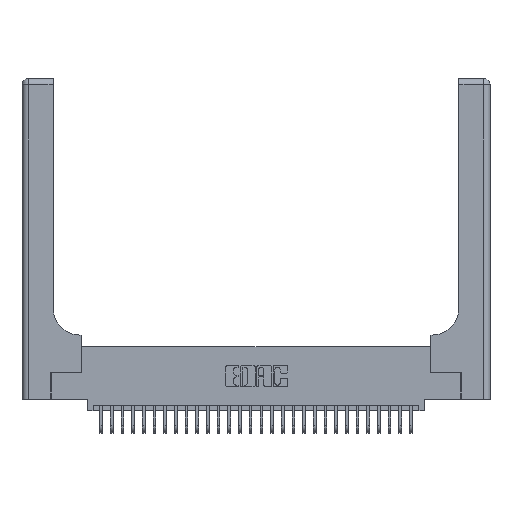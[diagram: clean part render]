
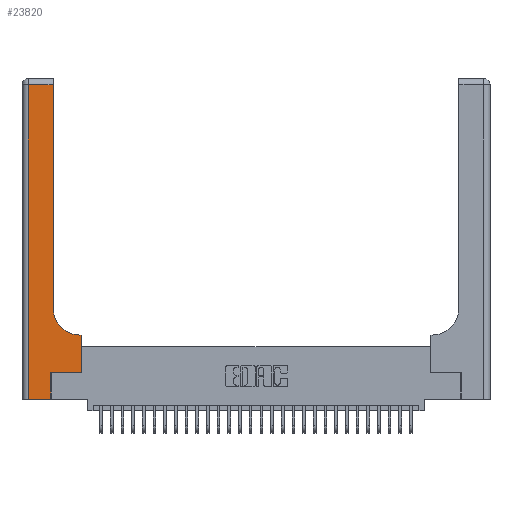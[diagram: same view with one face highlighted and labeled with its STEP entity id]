
A CAD part, top view. The second image highlights one B-rep face of the part: STEP entity #23820.
In plain terms, the highlighted planar face has unit normal (0, 0, 1).
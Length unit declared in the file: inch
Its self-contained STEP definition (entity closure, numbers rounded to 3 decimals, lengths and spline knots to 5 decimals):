
#377 = AXIS2_PLACEMENT_3D ( 'NONE', #19312, #4376, #21785 ) ;
#1062 = EDGE_CURVE ( 'NONE', #21715, #22190, #10786, .T. ) ;
#1196 = VECTOR ( 'NONE', #5113, 39.37008 ) ;
#1366 = EDGE_CURVE ( 'NONE', #31991, #13463, #16976, .T. ) ;
#1602 = CARTESIAN_POINT ( 'NONE',  ( 0.5415, 0.6, 0.37 ) ) ;
#2216 = VERTEX_POINT ( 'NONE', #30180 ) ;
#3138 = ORIENTED_EDGE ( 'NONE', *, *, #14814, .T. ) ;
#3196 = LINE ( 'NONE', #15899, #11464 ) ;
#3696 = VECTOR ( 'NONE', #29166, 39.37008 ) ;
#4099 = VECTOR ( 'NONE', #30759, 39.37008 ) ;
#4188 = EDGE_LOOP ( 'NONE', ( #12553, #32121, #7491, #20711, #28719, #3138, #16432, #11417, #30984 ) ) ;
#4376 = DIRECTION ( 'NONE',  ( 0., 0., -1. ) ) ;
#5113 = DIRECTION ( 'NONE',  ( -1., 0., 0. ) ) ;
#5179 = LINE ( 'NONE', #13146, #16843 ) ;
#6065 = DIRECTION ( 'NONE',  ( 1., 0., 0. ) ) ;
#6357 = CARTESIAN_POINT ( 'NONE',  ( 0.5585, 0.6, 0.37 ) ) ;
#7491 = ORIENTED_EDGE ( 'NONE', *, *, #1062, .T. ) ;
#7966 = LINE ( 'NONE', #27280, #1196 ) ;
#8907 = CARTESIAN_POINT ( 'NONE',  ( 0.2915, 2.94, 0.37 ) ) ;
#10083 = CARTESIAN_POINT ( 'NONE',  ( 0., 3., 0.37 ) ) ;
#10786 = LINE ( 'NONE', #13496, #4099 ) ;
#10850 = CARTESIAN_POINT ( 'NONE',  ( 0.5585, 0.25, 0.37 ) ) ;
#10950 = CARTESIAN_POINT ( 'NONE',  ( 0.2915, 3., 0.37 ) ) ;
#11417 = ORIENTED_EDGE ( 'NONE', *, *, #29906, .T. ) ;
#11464 = VECTOR ( 'NONE', #30570, 39.37008 ) ;
#11958 = CARTESIAN_POINT ( 'NONE',  ( 0.5585, 0.25, 0.37 ) ) ;
#12038 = EDGE_CURVE ( 'NONE', #2216, #28233, #3196, .T. ) ;
#12553 = ORIENTED_EDGE ( 'NONE', *, *, #23826, .T. ) ;
#12583 = DIRECTION ( 'NONE',  ( 0., 0., -1. ) ) ;
#12895 = VERTEX_POINT ( 'NONE', #1602 ) ;
#13128 = FACE_OUTER_BOUND ( 'NONE', #4188, .T. ) ;
#13146 = CARTESIAN_POINT ( 'NONE',  ( 0.269, 0.25, 0.37 ) ) ;
#13463 = VERTEX_POINT ( 'NONE', #6357 ) ;
#13496 = CARTESIAN_POINT ( 'NONE',  ( 0.06, 3., 0.37 ) ) ;
#13615 = CARTESIAN_POINT ( 'NONE',  ( 0., 2.94, 0.37 ) ) ;
#14814 = EDGE_CURVE ( 'NONE', #28233, #31991, #5179, .T. ) ;
#15082 = DIRECTION ( 'NONE',  ( 0., 1., 0. ) ) ;
#15899 = CARTESIAN_POINT ( 'NONE',  ( 0.269, 0., 0.37 ) ) ;
#16101 = DIRECTION ( 'NONE',  ( -1., 0., 0. ) ) ;
#16432 = ORIENTED_EDGE ( 'NONE', *, *, #1366, .T. ) ;
#16533 = VECTOR ( 'NONE', #16101, 39.37008 ) ;
#16843 = VECTOR ( 'NONE', #20636, 39.37008 ) ;
#16976 = LINE ( 'NONE', #11958, #3696 ) ;
#16995 = CARTESIAN_POINT ( 'NONE',  ( 0.06, 2.94, 0.37 ) ) ;
#17264 = CARTESIAN_POINT ( 'NONE',  ( 0.2915, 0.85, 0.37 ) ) ;
#18191 = VECTOR ( 'NONE', #6065, 39.37008 ) ;
#18557 = CARTESIAN_POINT ( 'NONE',  ( 0., 0., 0.37 ) ) ;
#19312 = CARTESIAN_POINT ( 'NONE',  ( 0.5415, 0.85, 0.37 ) ) ;
#19432 = CIRCLE ( 'NONE', #377, 0.25 ) ;
#19739 = LINE ( 'NONE', #10950, #25460 ) ;
#20230 = EDGE_CURVE ( 'NONE', #21026, #21715, #27308, .T. ) ;
#20636 = DIRECTION ( 'NONE',  ( 1., 0., 0. ) ) ;
#20711 = ORIENTED_EDGE ( 'NONE', *, *, #23418, .T. ) ;
#21026 = VERTEX_POINT ( 'NONE', #8907 ) ;
#21715 = VERTEX_POINT ( 'NONE', #16995 ) ;
#21785 = DIRECTION ( 'NONE',  ( 1., 0., 0. ) ) ;
#22190 = VERTEX_POINT ( 'NONE', #26207 ) ;
#23418 = EDGE_CURVE ( 'NONE', #22190, #2216, #25487, .T. ) ;
#23820 = ADVANCED_FACE ( 'NONE', ( #13128 ), #24870, .F. ) ;
#23826 = EDGE_CURVE ( 'NONE', #26527, #21026, #19739, .T. ) ;
#24870 = PLANE ( 'NONE',  #26456 ) ;
#25460 = VECTOR ( 'NONE', #15082, 39.37008 ) ;
#25487 = LINE ( 'NONE', #18557, #18191 ) ;
#25771 = CARTESIAN_POINT ( 'NONE',  ( 0.269, 0.25, 0.37 ) ) ;
#26207 = CARTESIAN_POINT ( 'NONE',  ( 0.06, 0., 0.37 ) ) ;
#26456 = AXIS2_PLACEMENT_3D ( 'NONE', #10083, #12583, #29778 ) ;
#26527 = VERTEX_POINT ( 'NONE', #17264 ) ;
#27096 = EDGE_CURVE ( 'NONE', #12895, #26527, #19432, .T. ) ;
#27280 = CARTESIAN_POINT ( 'NONE',  ( 0.2915, 0.6, 0.37 ) ) ;
#27308 = LINE ( 'NONE', #13615, #16533 ) ;
#28233 = VERTEX_POINT ( 'NONE', #25771 ) ;
#28719 = ORIENTED_EDGE ( 'NONE', *, *, #12038, .T. ) ;
#29166 = DIRECTION ( 'NONE',  ( 0., 1., 0. ) ) ;
#29778 = DIRECTION ( 'NONE',  ( -1., 0., 0. ) ) ;
#29906 = EDGE_CURVE ( 'NONE', #13463, #12895, #7966, .T. ) ;
#30180 = CARTESIAN_POINT ( 'NONE',  ( 0.269, 0., 0.37 ) ) ;
#30570 = DIRECTION ( 'NONE',  ( 0., 1., 0. ) ) ;
#30759 = DIRECTION ( 'NONE',  ( 0., -1., 0. ) ) ;
#30984 = ORIENTED_EDGE ( 'NONE', *, *, #27096, .T. ) ;
#31991 = VERTEX_POINT ( 'NONE', #10850 ) ;
#32121 = ORIENTED_EDGE ( 'NONE', *, *, #20230, .T. ) ;
